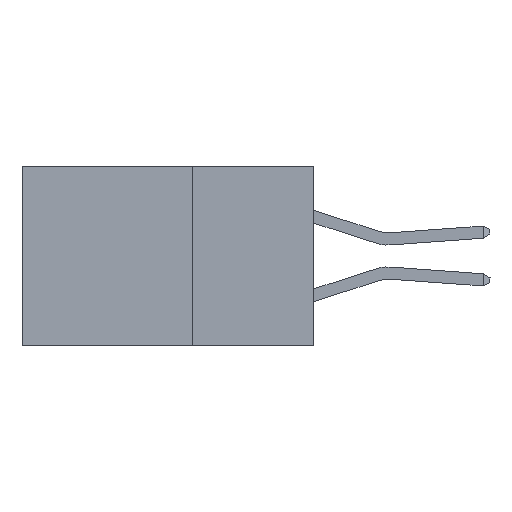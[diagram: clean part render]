
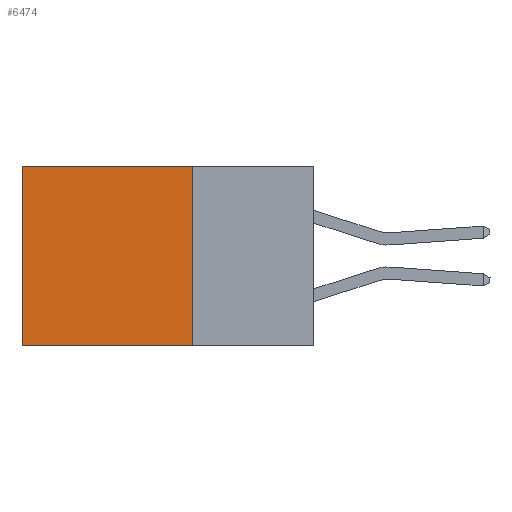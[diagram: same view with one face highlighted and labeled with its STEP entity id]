
A CAD part, left-side view. The second image highlights one B-rep face of the part: STEP entity #6474.
In plain terms, the highlighted planar face has unit normal (-1, 0, 0).
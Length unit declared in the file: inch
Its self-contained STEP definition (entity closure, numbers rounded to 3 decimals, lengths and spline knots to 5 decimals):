
#106 = LINE ( 'NONE', #11977, #8927 ) ;
#344 = PLANE ( 'NONE',  #842 ) ;
#415 = CARTESIAN_POINT ( 'NONE',  ( 0.2875, 0.25, 0. ) ) ;
#842 = AXIS2_PLACEMENT_3D ( 'NONE', #7953, #4698, #11219 ) ;
#1211 = ORIENTED_EDGE ( 'NONE', *, *, #10070, .T. ) ;
#1979 = ORIENTED_EDGE ( 'NONE', *, *, #9859, .T. ) ;
#2031 = CARTESIAN_POINT ( 'NONE',  ( 0.2875, 0.6, 0. ) ) ;
#3598 = DIRECTION ( 'NONE',  ( 0., 1., 0. ) ) ;
#4356 = LINE ( 'NONE', #12310, #12707 ) ;
#4585 = VERTEX_POINT ( 'NONE', #10275 ) ;
#4698 = DIRECTION ( 'NONE',  ( 1., 0., 0. ) ) ;
#5753 = VERTEX_POINT ( 'NONE', #12970 ) ;
#5792 = VERTEX_POINT ( 'NONE', #2031 ) ;
#6455 = EDGE_CURVE ( 'NONE', #4585, #5753, #13892, .T. ) ;
#6474 = ADVANCED_FACE ( 'NONE', ( #10985 ), #344, .F. ) ;
#6818 = DIRECTION ( 'NONE',  ( 0., 0., -1. ) ) ;
#6856 = EDGE_CURVE ( 'NONE', #11361, #4585, #106, .T. ) ;
#7452 = EDGE_LOOP ( 'NONE', ( #1211, #7712, #9963, #1979 ) ) ;
#7524 = DIRECTION ( 'NONE',  ( 0., 1., 0. ) ) ;
#7712 = ORIENTED_EDGE ( 'NONE', *, *, #6455, .F. ) ;
#7953 = CARTESIAN_POINT ( 'NONE',  ( 0.2875, 0.25, 0. ) ) ;
#8783 = VECTOR ( 'NONE', #3598, 39.37008 ) ;
#8927 = VECTOR ( 'NONE', #10817, 39.37008 ) ;
#9859 = EDGE_CURVE ( 'NONE', #11361, #5792, #11004, .T. ) ;
#9963 = ORIENTED_EDGE ( 'NONE', *, *, #6856, .F. ) ;
#10070 = EDGE_CURVE ( 'NONE', #5792, #5753, #4356, .T. ) ;
#10275 = CARTESIAN_POINT ( 'NONE',  ( 0.2875, 0.25, -0.37 ) ) ;
#10817 = DIRECTION ( 'NONE',  ( 0., 0., -1. ) ) ;
#10985 = FACE_OUTER_BOUND ( 'NONE', #7452, .T. ) ;
#11004 = LINE ( 'NONE', #11915, #11172 ) ;
#11172 = VECTOR ( 'NONE', #7524, 39.37008 ) ;
#11219 = DIRECTION ( 'NONE',  ( 0., 0., -1. ) ) ;
#11361 = VERTEX_POINT ( 'NONE', #415 ) ;
#11915 = CARTESIAN_POINT ( 'NONE',  ( 0.2875, 0.25, 0. ) ) ;
#11977 = CARTESIAN_POINT ( 'NONE',  ( 0.2875, 0.25, 0. ) ) ;
#12310 = CARTESIAN_POINT ( 'NONE',  ( 0.2875, 0.6, 0. ) ) ;
#12707 = VECTOR ( 'NONE', #6818, 39.37008 ) ;
#12970 = CARTESIAN_POINT ( 'NONE',  ( 0.2875, 0.6, -0.37 ) ) ;
#13468 = CARTESIAN_POINT ( 'NONE',  ( 0.2875, 0.25, -0.37 ) ) ;
#13892 = LINE ( 'NONE', #13468, #8783 ) ;
